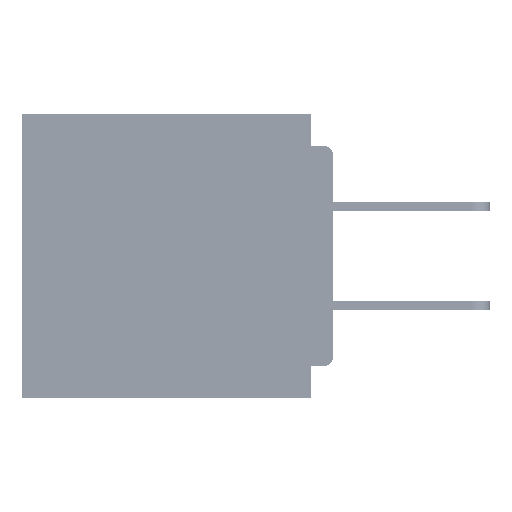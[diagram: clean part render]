
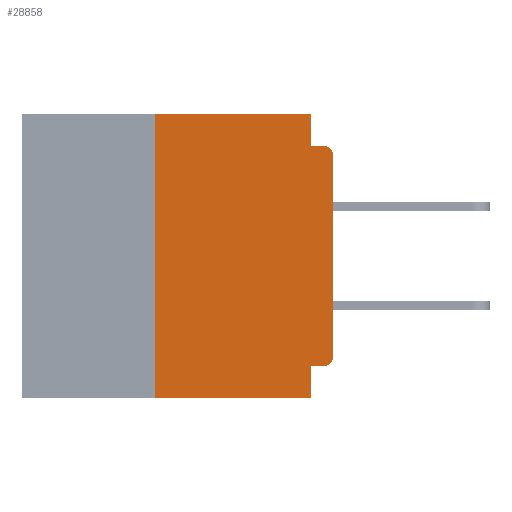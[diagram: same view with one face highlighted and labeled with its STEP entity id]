
A CAD part, left-side view. The second image highlights one B-rep face of the part: STEP entity #28858.
In plain terms, the highlighted planar face has unit normal (-1, 0, 0).
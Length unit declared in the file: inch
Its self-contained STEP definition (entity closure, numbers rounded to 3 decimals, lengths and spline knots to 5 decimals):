
#356 = CARTESIAN_POINT ( 'NONE',  ( 0., 0.25, -0.4 ) ) ;
#676 = FACE_OUTER_BOUND ( 'NONE', #49230, .T. ) ;
#2711 = LINE ( 'NONE', #22002, #28408 ) ;
#4037 = VERTEX_POINT ( 'NONE', #50499 ) ;
#5909 = CARTESIAN_POINT ( 'NONE',  ( 0., 0.25, 0. ) ) ;
#6612 = CARTESIAN_POINT ( 'NONE',  ( 0., 0., -0.045 ) ) ;
#6762 = DIRECTION ( 'NONE',  ( 0., -1., 0. ) ) ;
#6769 = LINE ( 'NONE', #61417, #18832 ) ;
#6891 = DIRECTION ( 'NONE',  ( 0., 0., 1. ) ) ;
#7697 = EDGE_CURVE ( 'NONE', #17375, #36387, #52663, .T. ) ;
#8998 = AXIS2_PLACEMENT_3D ( 'NONE', #19919, #55750, #25102 ) ;
#9531 = EDGE_CURVE ( 'NONE', #36387, #4037, #29161, .T. ) ;
#9609 = PLANE ( 'NONE',  #8998 ) ;
#9829 = DIRECTION ( 'NONE',  ( -1., 0., 0. ) ) ;
#10681 = CARTESIAN_POINT ( 'NONE',  ( 0., 0.437, -0.4 ) ) ;
#12104 = VERTEX_POINT ( 'NONE', #42887 ) ;
#14428 = CIRCLE ( 'NONE', #19714, 0.015 ) ;
#15533 = VECTOR ( 'NONE', #22102, 39.37008 ) ;
#16369 = ORIENTED_EDGE ( 'NONE', *, *, #40149, .T. ) ;
#16747 = CARTESIAN_POINT ( 'NONE',  ( 0., 0., -0.34 ) ) ;
#16858 = DIRECTION ( 'NONE',  ( 0., 1., 0. ) ) ;
#17010 = CARTESIAN_POINT ( 'NONE',  ( 0., 0.25, -0.4 ) ) ;
#17167 = CARTESIAN_POINT ( 'NONE',  ( 0., 0.031, 0. ) ) ;
#17375 = VERTEX_POINT ( 'NONE', #44083 ) ;
#17725 = VERTEX_POINT ( 'NONE', #5909 ) ;
#18832 = VECTOR ( 'NONE', #51122, 39.37008 ) ;
#19714 = AXIS2_PLACEMENT_3D ( 'NONE', #26018, #61798, #31156 ) ;
#19919 = CARTESIAN_POINT ( 'NONE',  ( 0., 0.437, 0. ) ) ;
#20526 = ORIENTED_EDGE ( 'NONE', *, *, #20677, .T. ) ;
#20677 = EDGE_CURVE ( 'NONE', #12104, #4037, #61837, .T. ) ;
#21237 = ORIENTED_EDGE ( 'NONE', *, *, #9531, .F. ) ;
#22002 = CARTESIAN_POINT ( 'NONE',  ( 0., 0., -0.355 ) ) ;
#22102 = DIRECTION ( 'NONE',  ( 0., -1., 0. ) ) ;
#22308 = DIRECTION ( 'NONE',  ( 0., 0., -1. ) ) ;
#23573 = ORIENTED_EDGE ( 'NONE', *, *, #7697, .F. ) ;
#25102 = DIRECTION ( 'NONE',  ( 0., 0., -1. ) ) ;
#25437 = EDGE_CURVE ( 'NONE', #17725, #17375, #30071, .T. ) ;
#26018 = CARTESIAN_POINT ( 'NONE',  ( 0., 0.015, -0.34 ) ) ;
#27737 = ORIENTED_EDGE ( 'NONE', *, *, #25437, .F. ) ;
#28031 = EDGE_CURVE ( 'NONE', #53462, #40160, #14428, .T. ) ;
#28408 = VECTOR ( 'NONE', #16858, 39.37008 ) ;
#28474 = VECTOR ( 'NONE', #6762, 39.37008 ) ;
#28571 = ORIENTED_EDGE ( 'NONE', *, *, #53789, .F. ) ;
#28709 = VERTEX_POINT ( 'NONE', #356 ) ;
#28713 = EDGE_CURVE ( 'NONE', #28709, #61466, #64777, .T. ) ;
#28858 = ADVANCED_FACE ( 'NONE', ( #676 ), #9609, .F. ) ;
#29161 = LINE ( 'NONE', #6612, #15533 ) ;
#30071 = LINE ( 'NONE', #32337, #28474 ) ;
#30488 = LINE ( 'NONE', #17010, #45729 ) ;
#31156 = DIRECTION ( 'NONE',  ( 0., 0., -1. ) ) ;
#32337 = CARTESIAN_POINT ( 'NONE',  ( 0., 0.437, 0. ) ) ;
#34107 = ORIENTED_EDGE ( 'NONE', *, *, #28713, .T. ) ;
#35691 = ORIENTED_EDGE ( 'NONE', *, *, #48696, .F. ) ;
#36122 = VERTEX_POINT ( 'NONE', #39669 ) ;
#36387 = VERTEX_POINT ( 'NONE', #46790 ) ;
#36527 = ORIENTED_EDGE ( 'NONE', *, *, #50663, .F. ) ;
#39669 = CARTESIAN_POINT ( 'NONE',  ( 0., 0.031, -0.355 ) ) ;
#40149 = EDGE_CURVE ( 'NONE', #40160, #12104, #63159, .T. ) ;
#40160 = VERTEX_POINT ( 'NONE', #16747 ) ;
#40577 = CARTESIAN_POINT ( 'NONE',  ( 0., 0.015, -0.06 ) ) ;
#42294 = CARTESIAN_POINT ( 'NONE',  ( 0., 0., 0. ) ) ;
#42845 = ORIENTED_EDGE ( 'NONE', *, *, #28031, .T. ) ;
#42887 = CARTESIAN_POINT ( 'NONE',  ( 0., 0., -0.06 ) ) ;
#43895 = VECTOR ( 'NONE', #22308, 39.37008 ) ;
#44083 = CARTESIAN_POINT ( 'NONE',  ( 0., 0.031, 0. ) ) ;
#45697 = DIRECTION ( 'NONE',  ( 0., 0., -1. ) ) ;
#45729 = VECTOR ( 'NONE', #6891, 39.37008 ) ;
#46790 = CARTESIAN_POINT ( 'NONE',  ( 0., 0.031, -0.045 ) ) ;
#47432 = DIRECTION ( 'NONE',  ( 0., 0., 1. ) ) ;
#48696 = EDGE_CURVE ( 'NONE', #36122, #61466, #6769, .T. ) ;
#49230 = EDGE_LOOP ( 'NONE', ( #16369, #20526, #21237, #23573, #27737, #28571, #34107, #35691, #36527, #42845 ) ) ;
#50151 = CARTESIAN_POINT ( 'NONE',  ( 0., 0.015, -0.355 ) ) ;
#50499 = CARTESIAN_POINT ( 'NONE',  ( 0., 0.015, -0.045 ) ) ;
#50663 = EDGE_CURVE ( 'NONE', #53462, #36122, #2711, .T. ) ;
#51122 = DIRECTION ( 'NONE',  ( 0., 0., -1. ) ) ;
#51206 = VECTOR ( 'NONE', #51887, 39.37008 ) ;
#51887 = DIRECTION ( 'NONE',  ( 0., -1., 0. ) ) ;
#52663 = LINE ( 'NONE', #17167, #43895 ) ;
#53462 = VERTEX_POINT ( 'NONE', #50151 ) ;
#53789 = EDGE_CURVE ( 'NONE', #28709, #17725, #30488, .T. ) ;
#55750 = DIRECTION ( 'NONE',  ( 1., 0., 0. ) ) ;
#60271 = AXIS2_PLACEMENT_3D ( 'NONE', #40577, #9829, #45697 ) ;
#60864 = CARTESIAN_POINT ( 'NONE',  ( 0., 0.031, -0.4 ) ) ;
#61417 = CARTESIAN_POINT ( 'NONE',  ( 0., 0.031, -0.4 ) ) ;
#61466 = VERTEX_POINT ( 'NONE', #60864 ) ;
#61570 = VECTOR ( 'NONE', #47432, 39.37008 ) ;
#61798 = DIRECTION ( 'NONE',  ( -1., 0., 0. ) ) ;
#61837 = CIRCLE ( 'NONE', #60271, 0.015 ) ;
#63159 = LINE ( 'NONE', #42294, #61570 ) ;
#64777 = LINE ( 'NONE', #10681, #51206 ) ;
